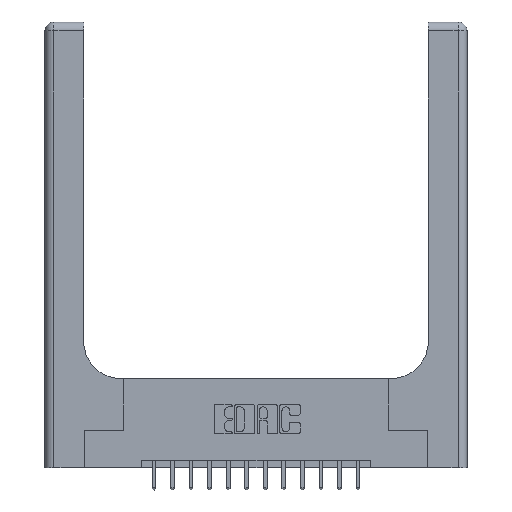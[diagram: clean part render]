
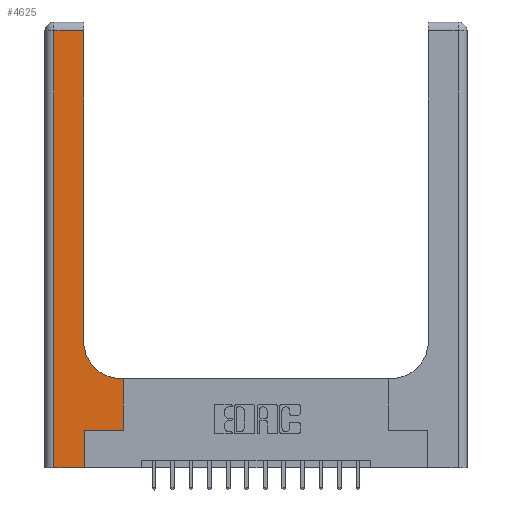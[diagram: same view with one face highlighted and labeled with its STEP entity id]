
A CAD part, top view. The second image highlights one B-rep face of the part: STEP entity #4625.
In plain terms, the highlighted planar face has unit normal (0, 0, 1).
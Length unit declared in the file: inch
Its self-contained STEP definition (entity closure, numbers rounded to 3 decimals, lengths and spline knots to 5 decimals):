
#3 = VERTEX_POINT ( 'NONE', #13697 ) ;
#127 = DIRECTION ( 'NONE',  ( -1., 0., 0. ) ) ;
#947 = DIRECTION ( 'NONE',  ( 1., 0., 0. ) ) ;
#1127 = LINE ( 'NONE', #14913, #16426 ) ;
#1452 = DIRECTION ( 'NONE',  ( 0., 1., 0. ) ) ;
#1630 = EDGE_CURVE ( 'NONE', #11090, #3976, #13684, .T. ) ;
#1644 = VERTEX_POINT ( 'NONE', #12714 ) ;
#2324 = LINE ( 'NONE', #8001, #5633 ) ;
#2341 = ORIENTED_EDGE ( 'NONE', *, *, #10795, .T. ) ;
#2349 = DIRECTION ( 'NONE',  ( -1., 0., 0. ) ) ;
#2408 = LINE ( 'NONE', #3577, #16073 ) ;
#2471 = CARTESIAN_POINT ( 'NONE',  ( 0., 3., 0.37 ) ) ;
#2473 = DIRECTION ( 'NONE',  ( -1., 0., 0. ) ) ;
#2771 = VERTEX_POINT ( 'NONE', #12562 ) ;
#3052 = EDGE_CURVE ( 'NONE', #3183, #11090, #9885, .T. ) ;
#3183 = VERTEX_POINT ( 'NONE', #5699 ) ;
#3286 = DIRECTION ( 'NONE',  ( 1., 0., 0. ) ) ;
#3577 = CARTESIAN_POINT ( 'NONE',  ( 0.265, 0.25, 0.37 ) ) ;
#3876 = EDGE_CURVE ( 'NONE', #2771, #10089, #2408, .T. ) ;
#3976 = VERTEX_POINT ( 'NONE', #6012 ) ;
#4223 = LINE ( 'NONE', #16599, #11687 ) ;
#4357 = DIRECTION ( 'NONE',  ( 0., -1., 0. ) ) ;
#4463 = CARTESIAN_POINT ( 'NONE',  ( 0.51, 0.6, 0.37 ) ) ;
#4558 = DIRECTION ( 'NONE',  ( 0., 0., -1. ) ) ;
#4625 = ADVANCED_FACE ( 'NONE', ( #6920 ), #11787, .F. ) ;
#5112 = VERTEX_POINT ( 'NONE', #4463 ) ;
#5349 = DIRECTION ( 'NONE',  ( 0., 0., -1. ) ) ;
#5633 = VECTOR ( 'NONE', #9386, 39.37008 ) ;
#5699 = CARTESIAN_POINT ( 'NONE',  ( 0.26, 0.85, 0.37 ) ) ;
#6012 = CARTESIAN_POINT ( 'NONE',  ( 0.06, 2.94, 0.37 ) ) ;
#6920 = FACE_OUTER_BOUND ( 'NONE', #7975, .T. ) ;
#6983 = EDGE_CURVE ( 'NONE', #3976, #7751, #1127, .T. ) ;
#7202 = ORIENTED_EDGE ( 'NONE', *, *, #15063, .T. ) ;
#7402 = CARTESIAN_POINT ( 'NONE',  ( 0.26, 2.94, 0.37 ) ) ;
#7567 = EDGE_CURVE ( 'NONE', #3, #2771, #2324, .T. ) ;
#7751 = VERTEX_POINT ( 'NONE', #9554 ) ;
#7903 = CARTESIAN_POINT ( 'NONE',  ( 0.26, 3., 0.37 ) ) ;
#7958 = ORIENTED_EDGE ( 'NONE', *, *, #3052, .T. ) ;
#7975 = EDGE_LOOP ( 'NONE', ( #7958, #15243, #15843, #14336, #14088, #10881, #7202, #2341, #16661 ) ) ;
#8001 = CARTESIAN_POINT ( 'NONE',  ( 0.265, 0., 0.37 ) ) ;
#8275 = CARTESIAN_POINT ( 'NONE',  ( 0.528, 0.25, 0.37 ) ) ;
#8362 = AXIS2_PLACEMENT_3D ( 'NONE', #2471, #5349, #127 ) ;
#8443 = LINE ( 'NONE', #13021, #10284 ) ;
#9386 = DIRECTION ( 'NONE',  ( 0., 1., 0. ) ) ;
#9554 = CARTESIAN_POINT ( 'NONE',  ( 0.06, 0., 0.37 ) ) ;
#9885 = LINE ( 'NONE', #7903, #16298 ) ;
#10089 = VERTEX_POINT ( 'NONE', #14058 ) ;
#10284 = VECTOR ( 'NONE', #2473, 39.37008 ) ;
#10795 = EDGE_CURVE ( 'NONE', #1644, #5112, #8443, .T. ) ;
#10881 = ORIENTED_EDGE ( 'NONE', *, *, #3876, .T. ) ;
#11090 = VERTEX_POINT ( 'NONE', #7402 ) ;
#11285 = LINE ( 'NONE', #8275, #15208 ) ;
#11385 = CARTESIAN_POINT ( 'NONE',  ( 0., 2.94, 0.37 ) ) ;
#11396 = VECTOR ( 'NONE', #2349, 39.37008 ) ;
#11687 = VECTOR ( 'NONE', #16541, 39.37008 ) ;
#11787 = PLANE ( 'NONE',  #8362 ) ;
#12507 = CARTESIAN_POINT ( 'NONE',  ( 0.51, 0.85, 0.37 ) ) ;
#12545 = EDGE_CURVE ( 'NONE', #7751, #3, #4223, .T. ) ;
#12562 = CARTESIAN_POINT ( 'NONE',  ( 0.265, 0.25, 0.37 ) ) ;
#12714 = CARTESIAN_POINT ( 'NONE',  ( 0.528, 0.6, 0.37 ) ) ;
#13021 = CARTESIAN_POINT ( 'NONE',  ( 0.26, 0.6, 0.37 ) ) ;
#13684 = LINE ( 'NONE', #11385, #11396 ) ;
#13697 = CARTESIAN_POINT ( 'NONE',  ( 0.265, 0., 0.37 ) ) ;
#14058 = CARTESIAN_POINT ( 'NONE',  ( 0.528, 0.25, 0.37 ) ) ;
#14088 = ORIENTED_EDGE ( 'NONE', *, *, #7567, .T. ) ;
#14336 = ORIENTED_EDGE ( 'NONE', *, *, #12545, .T. ) ;
#14398 = CIRCLE ( 'NONE', #15668, 0.25 ) ;
#14828 = DIRECTION ( 'NONE',  ( 0., 1., 0. ) ) ;
#14913 = CARTESIAN_POINT ( 'NONE',  ( 0.06, 3., 0.37 ) ) ;
#15063 = EDGE_CURVE ( 'NONE', #10089, #1644, #11285, .T. ) ;
#15194 = EDGE_CURVE ( 'NONE', #5112, #3183, #14398, .T. ) ;
#15208 = VECTOR ( 'NONE', #14828, 39.37008 ) ;
#15243 = ORIENTED_EDGE ( 'NONE', *, *, #1630, .T. ) ;
#15668 = AXIS2_PLACEMENT_3D ( 'NONE', #12507, #4558, #3286 ) ;
#15843 = ORIENTED_EDGE ( 'NONE', *, *, #6983, .T. ) ;
#16073 = VECTOR ( 'NONE', #947, 39.37008 ) ;
#16298 = VECTOR ( 'NONE', #1452, 39.37008 ) ;
#16426 = VECTOR ( 'NONE', #4357, 39.37008 ) ;
#16541 = DIRECTION ( 'NONE',  ( 1., 0., 0. ) ) ;
#16599 = CARTESIAN_POINT ( 'NONE',  ( 0., 0., 0.37 ) ) ;
#16661 = ORIENTED_EDGE ( 'NONE', *, *, #15194, .T. ) ;
